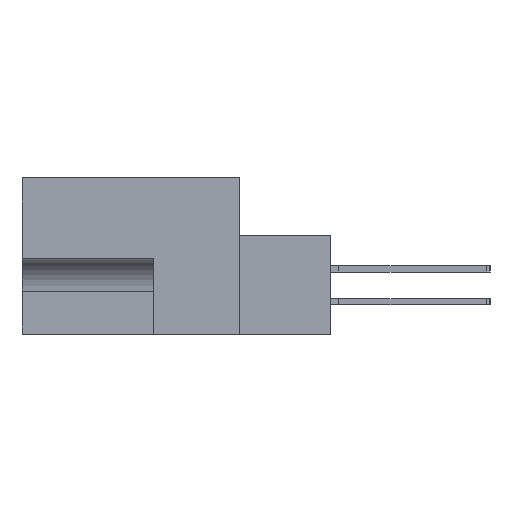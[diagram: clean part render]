
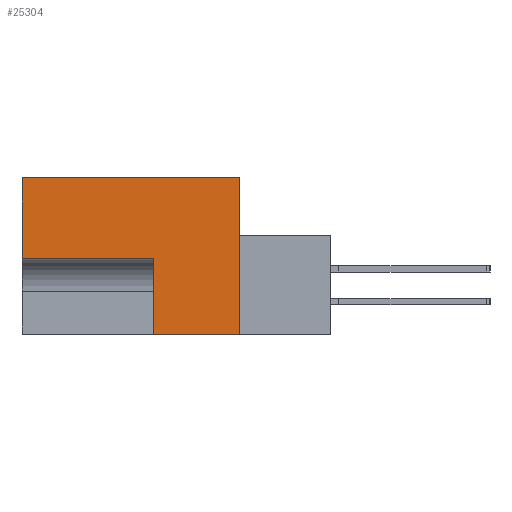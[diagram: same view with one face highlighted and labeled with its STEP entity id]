
A CAD part, left-side view. The second image highlights one B-rep face of the part: STEP entity #25304.
In plain terms, the highlighted planar face has unit normal (-1, 0, 0).
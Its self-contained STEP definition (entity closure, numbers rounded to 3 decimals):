
#1593 = VERTEX_POINT ( 'NONE', #46104 ) ;
#3322 = VECTOR ( 'NONE', #44170, 1000. ) ;
#4777 = EDGE_LOOP ( 'NONE', ( #17221, #10463, #35114, #38910, #12192, #22449 ) ) ;
#5434 = CARTESIAN_POINT ( 'NONE',  ( 0., 0., 0. ) ) ;
#7048 = VECTOR ( 'NONE', #44880, 1000. ) ;
#7050 = CARTESIAN_POINT ( 'NONE',  ( 0., 20.955, 0. ) ) ;
#8704 = DIRECTION ( 'NONE',  ( 0., -1., 0. ) ) ;
#8754 = VECTOR ( 'NONE', #31115, 1000. ) ;
#10463 = ORIENTED_EDGE ( 'NONE', *, *, #26489, .F. ) ;
#10889 = CARTESIAN_POINT ( 'NONE',  ( 0., 8.255, -15.088 ) ) ;
#11539 = CARTESIAN_POINT ( 'NONE',  ( 0., 8.255, -7.772 ) ) ;
#12192 = ORIENTED_EDGE ( 'NONE', *, *, #13428, .F. ) ;
#12532 = CARTESIAN_POINT ( 'NONE',  ( 0., 0., 0. ) ) ;
#13428 = EDGE_CURVE ( 'NONE', #27466, #26497, #32468, .T. ) ;
#15604 = CARTESIAN_POINT ( 'NONE',  ( 0., 0., -15.088 ) ) ;
#17221 = ORIENTED_EDGE ( 'NONE', *, *, #48284, .F. ) ;
#18191 = PLANE ( 'NONE',  #34486 ) ;
#18763 = EDGE_CURVE ( 'NONE', #41671, #1593, #38900, .T. ) ;
#20598 = CARTESIAN_POINT ( 'NONE',  ( 0., 11.506, 0. ) ) ;
#21121 = VERTEX_POINT ( 'NONE', #15604 ) ;
#22020 = DIRECTION ( 'NONE',  ( 1., 0., 0. ) ) ;
#22449 = ORIENTED_EDGE ( 'NONE', *, *, #37581, .F. ) ;
#23264 = LINE ( 'NONE', #29444, #7048 ) ;
#25304 = ADVANCED_FACE ( 'NONE', ( #48474 ), #18191, .F. ) ;
#26489 = EDGE_CURVE ( 'NONE', #1593, #21121, #35141, .T. ) ;
#26497 = VERTEX_POINT ( 'NONE', #40633 ) ;
#27466 = VERTEX_POINT ( 'NONE', #11539 ) ;
#29444 = CARTESIAN_POINT ( 'NONE',  ( 0., -8.814, -15.088 ) ) ;
#29896 = VECTOR ( 'NONE', #39761, 1000. ) ;
#31115 = DIRECTION ( 'NONE',  ( 0., 0., 1. ) ) ;
#31218 = LINE ( 'NONE', #10889, #8754 ) ;
#32468 = LINE ( 'NONE', #48564, #29896 ) ;
#34217 = LINE ( 'NONE', #37483, #34805 ) ;
#34486 = AXIS2_PLACEMENT_3D ( 'NONE', #5434, #22020, #37377 ) ;
#34805 = VECTOR ( 'NONE', #41695, 1000. ) ;
#35114 = ORIENTED_EDGE ( 'NONE', *, *, #18763, .F. ) ;
#35141 = LINE ( 'NONE', #12532, #3322 ) ;
#37377 = DIRECTION ( 'NONE',  ( 0., 0., -1. ) ) ;
#37483 = CARTESIAN_POINT ( 'NONE',  ( 0., 20.955, -15.088 ) ) ;
#37581 = EDGE_CURVE ( 'NONE', #44863, #27466, #31218, .T. ) ;
#38900 = LINE ( 'NONE', #20598, #51473 ) ;
#38910 = ORIENTED_EDGE ( 'NONE', *, *, #39425, .F. ) ;
#39425 = EDGE_CURVE ( 'NONE', #26497, #41671, #34217, .T. ) ;
#39761 = DIRECTION ( 'NONE',  ( 0., 1., 0. ) ) ;
#40633 = CARTESIAN_POINT ( 'NONE',  ( 0., 20.955, -7.772 ) ) ;
#41434 = CARTESIAN_POINT ( 'NONE',  ( 0., 8.255, -15.088 ) ) ;
#41671 = VERTEX_POINT ( 'NONE', #7050 ) ;
#41695 = DIRECTION ( 'NONE',  ( 0., 0., 1. ) ) ;
#44170 = DIRECTION ( 'NONE',  ( 0., 0., -1. ) ) ;
#44863 = VERTEX_POINT ( 'NONE', #41434 ) ;
#44880 = DIRECTION ( 'NONE',  ( 0., 1., 0. ) ) ;
#46104 = CARTESIAN_POINT ( 'NONE',  ( 0., 0., 0. ) ) ;
#48284 = EDGE_CURVE ( 'NONE', #21121, #44863, #23264, .T. ) ;
#48474 = FACE_OUTER_BOUND ( 'NONE', #4777, .T. ) ;
#48564 = CARTESIAN_POINT ( 'NONE',  ( 0., 8.255, -7.772 ) ) ;
#51473 = VECTOR ( 'NONE', #8704, 1000. ) ;
